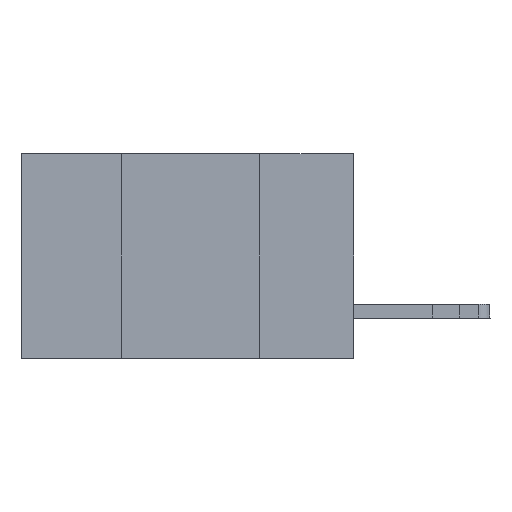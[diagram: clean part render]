
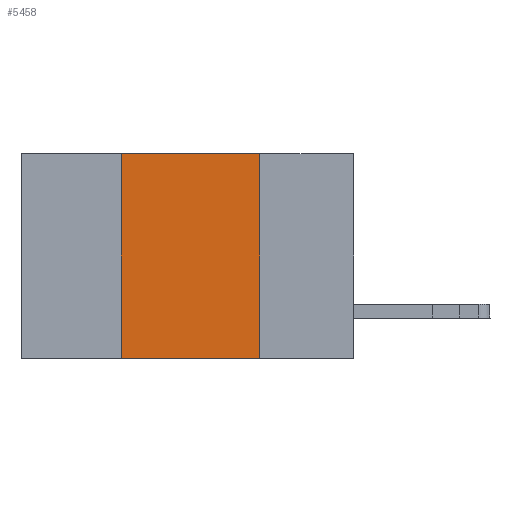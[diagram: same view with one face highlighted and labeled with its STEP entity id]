
A CAD part, left-side view. The second image highlights one B-rep face of the part: STEP entity #5458.
In plain terms, the highlighted planar face has unit normal (-1, 0, 0).
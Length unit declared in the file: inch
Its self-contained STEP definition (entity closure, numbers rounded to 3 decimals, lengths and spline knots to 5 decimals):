
#723 = EDGE_LOOP ( 'NONE', ( #7190, #2265, #13080, #13074 ) ) ;
#1078 = PLANE ( 'NONE',  #15211 ) ;
#1554 = FACE_OUTER_BOUND ( 'NONE', #723, .T. ) ;
#2265 = ORIENTED_EDGE ( 'NONE', *, *, #10072, .F. ) ;
#2927 = DIRECTION ( 'NONE',  ( 0., 0., -1. ) ) ;
#3072 = DIRECTION ( 'NONE',  ( 0., 0., 1. ) ) ;
#4680 = VERTEX_POINT ( 'NONE', #20487 ) ;
#5075 = LINE ( 'NONE', #19101, #10034 ) ;
#5458 = ADVANCED_FACE ( 'NONE', ( #1554 ), #1078, .F. ) ;
#6085 = CARTESIAN_POINT ( 'NONE',  ( 0., 0.6, -0.37 ) ) ;
#6196 = CARTESIAN_POINT ( 'NONE',  ( 0., 0.42, -0.37 ) ) ;
#7190 = ORIENTED_EDGE ( 'NONE', *, *, #16617, .F. ) ;
#7208 = CARTESIAN_POINT ( 'NONE',  ( 0., 0.42, 0. ) ) ;
#10034 = VECTOR ( 'NONE', #15530, 39.37008 ) ;
#10072 = EDGE_CURVE ( 'NONE', #14989, #12106, #20611, .T. ) ;
#10603 = CARTESIAN_POINT ( 'NONE',  ( 0., 0.6, 0. ) ) ;
#11955 = LINE ( 'NONE', #6085, #12528 ) ;
#12106 = VERTEX_POINT ( 'NONE', #20019 ) ;
#12528 = VECTOR ( 'NONE', #18887, 39.37008 ) ;
#13074 = ORIENTED_EDGE ( 'NONE', *, *, #21910, .T. ) ;
#13080 = ORIENTED_EDGE ( 'NONE', *, *, #21466, .F. ) ;
#13985 = DIRECTION ( 'NONE',  ( 1., 0., 0. ) ) ;
#14989 = VERTEX_POINT ( 'NONE', #7208 ) ;
#15211 = AXIS2_PLACEMENT_3D ( 'NONE', #22920, #13985, #2927 ) ;
#15239 = VECTOR ( 'NONE', #21449, 39.37008 ) ;
#15285 = VERTEX_POINT ( 'NONE', #6196 ) ;
#15530 = DIRECTION ( 'NONE',  ( 0., 0., -1. ) ) ;
#16617 = EDGE_CURVE ( 'NONE', #12106, #4680, #5075, .T. ) ;
#18887 = DIRECTION ( 'NONE',  ( 0., -1., 0. ) ) ;
#19101 = CARTESIAN_POINT ( 'NONE',  ( 0., 0.17, 0. ) ) ;
#20019 = CARTESIAN_POINT ( 'NONE',  ( 0., 0.17, 0. ) ) ;
#20487 = CARTESIAN_POINT ( 'NONE',  ( 0., 0.17, -0.37 ) ) ;
#20611 = LINE ( 'NONE', #10603, #15239 ) ;
#21284 = CARTESIAN_POINT ( 'NONE',  ( 0., 0.42, 0. ) ) ;
#21449 = DIRECTION ( 'NONE',  ( 0., -1., 0. ) ) ;
#21466 = EDGE_CURVE ( 'NONE', #15285, #14989, #22701, .T. ) ;
#21601 = VECTOR ( 'NONE', #3072, 39.37008 ) ;
#21910 = EDGE_CURVE ( 'NONE', #15285, #4680, #11955, .T. ) ;
#22701 = LINE ( 'NONE', #21284, #21601 ) ;
#22920 = CARTESIAN_POINT ( 'NONE',  ( 0., 0.6, 0. ) ) ;
